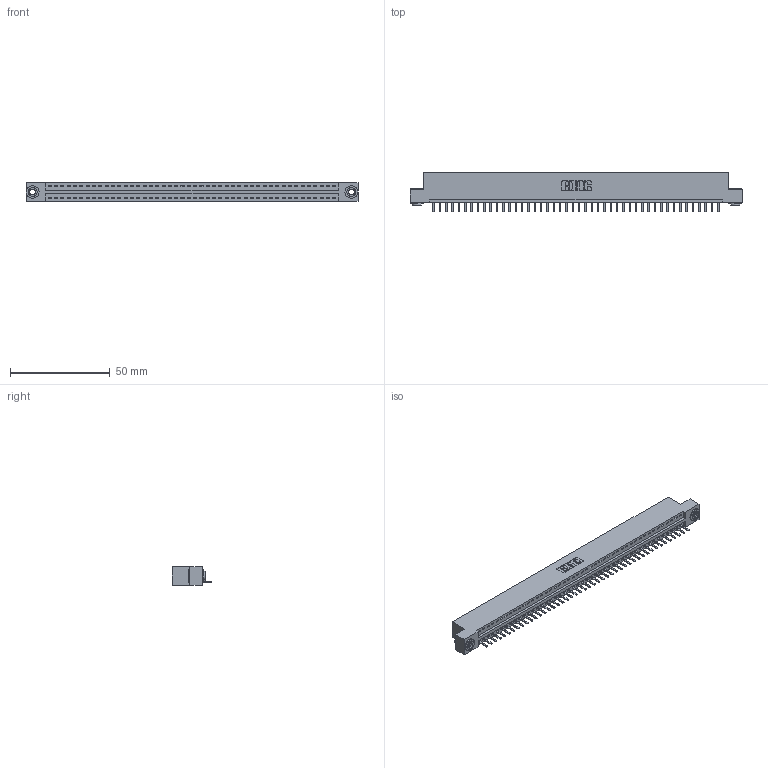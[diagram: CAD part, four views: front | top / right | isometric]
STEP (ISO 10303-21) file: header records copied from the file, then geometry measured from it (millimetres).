
FILE_DESCRIPTION (( 'STEP AP203' ), '1' );
FILE_NAME ('396-046-520-103.STEP', '2019-10-28T03:02:00', ( '' ), ( '' ), 'SwSTEP 2.0', 'SolidWorks 2016', '' );
FILE_SCHEMA (( 'CONFIG_CONTROL_DESIGN' ));
Length unit declared in the file: inch
Products named in the file (4): 345-292-001_345-293-120; 346 Part_Flush Mounting Lugs - 0.156 Dia-TH; 396-046-520-103; 345-250-002_345-250-002-102
Assembly tree (49 placements, depth 2):
  396-046-520-103
    346 Part_Flush Mounting Lugs - 0.156 Dia-TH
    345-292-001_345-293-120  x46
    345-250-002_345-250-002-102  x2
Bounding box: 166.62 x 20.02 x 9.4 mm (x, y, z)
Volume: 15864.2 mm3; surface area: 19648.9 mm2
Topology: 49 solids, 49 shells, 3012 faces, 8869 edges, 5786 vertices
Faces by surface type: plane 2018, cylinder 986, cone 8
Entity records: 28774 total; most frequent: CARTESIAN_POINT 4921, ORIENTED_EDGE 4882, DIRECTION 4355, EDGE_CURVE 2441, LINE 2097, VECTOR 2097, VERTEX_POINT 1622, AXIS2_PLACEMENT_3D 1129
